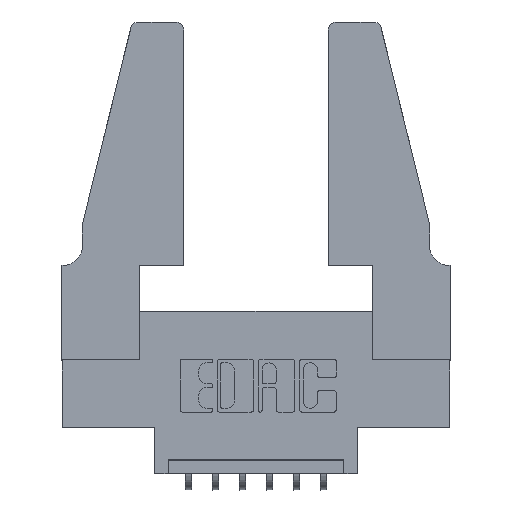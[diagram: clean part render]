
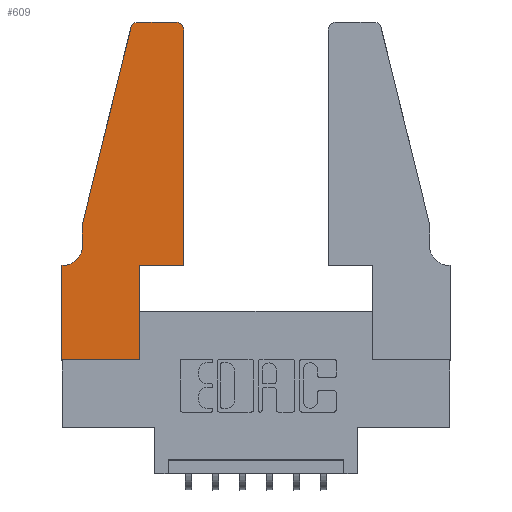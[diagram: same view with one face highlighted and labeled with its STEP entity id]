
A CAD part, top view. The second image highlights one B-rep face of the part: STEP entity #609.
In plain terms, the highlighted planar face has unit normal (0, 0, 1).
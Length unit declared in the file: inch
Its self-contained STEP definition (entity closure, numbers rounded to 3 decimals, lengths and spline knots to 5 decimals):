
#245 = EDGE_LOOP ( 'NONE', ( #11382, #3693, #6734, #3496, #2989, #1678, #5615, #2025, #9772, #2973, #2548, #9526 ) ) ;
#329 = VECTOR ( 'NONE', #9058, 39.37008 ) ;
#408 = LINE ( 'NONE', #6901, #4360 ) ;
#581 = CARTESIAN_POINT ( 'NONE',  ( 0.25487, 1.22718, 0.37 ) ) ;
#609 = ADVANCED_FACE ( 'NONE', ( #11190 ), #1291, .T. ) ;
#1291 = PLANE ( 'NONE',  #3030 ) ;
#1590 = VECTOR ( 'NONE', #2606, 39.37008 ) ;
#1604 = VERTEX_POINT ( 'NONE', #581 ) ;
#1656 = LINE ( 'NONE', #6720, #11586 ) ;
#1660 = CARTESIAN_POINT ( 'NONE',  ( 0.2605, 1.25, 0.37 ) ) ;
#1678 = ORIENTED_EDGE ( 'NONE', *, *, #3053, .T. ) ;
#1736 = LINE ( 'NONE', #8917, #1590 ) ;
#1852 = AXIS2_PLACEMENT_3D ( 'NONE', #11717, #9952, #9148 ) ;
#1861 = VERTEX_POINT ( 'NONE', #5412 ) ;
#2025 = ORIENTED_EDGE ( 'NONE', *, *, #3757, .T. ) ;
#2342 = EDGE_CURVE ( 'NONE', #1604, #7758, #8015, .T. ) ;
#2347 = CARTESIAN_POINT ( 'NONE',  ( 0.0755, 0.5, 0.37 ) ) ;
#2548 = ORIENTED_EDGE ( 'NONE', *, *, #7312, .T. ) ;
#2557 = CIRCLE ( 'NONE', #1852, 0.03 ) ;
#2606 = DIRECTION ( 'NONE',  ( 0., -1., 0. ) ) ;
#2674 = EDGE_CURVE ( 'NONE', #2938, #1604, #8461, .T. ) ;
#2734 = LINE ( 'NONE', #8519, #11380 ) ;
#2938 = VERTEX_POINT ( 'NONE', #3690 ) ;
#2939 = VECTOR ( 'NONE', #11372, 39.37008 ) ;
#2973 = ORIENTED_EDGE ( 'NONE', *, *, #9862, .T. ) ;
#2989 = ORIENTED_EDGE ( 'NONE', *, *, #3517, .T. ) ;
#3003 = DIRECTION ( 'NONE',  ( -1., 0., 0. ) ) ;
#3009 = DIRECTION ( 'NONE',  ( 0., 0., 1. ) ) ;
#3030 = AXIS2_PLACEMENT_3D ( 'NONE', #4083, #3009, #4995 ) ;
#3040 = DIRECTION ( 'NONE',  ( 0., -1., 0. ) ) ;
#3053 = EDGE_CURVE ( 'NONE', #10348, #5704, #9638, .T. ) ;
#3066 = DIRECTION ( 'NONE',  ( 1., 0., 0. ) ) ;
#3261 = LINE ( 'NONE', #4253, #11180 ) ;
#3496 = ORIENTED_EDGE ( 'NONE', *, *, #3575, .T. ) ;
#3517 = EDGE_CURVE ( 'NONE', #9332, #10348, #6536, .T. ) ;
#3575 = EDGE_CURVE ( 'NONE', #7758, #9332, #1656, .T. ) ;
#3690 = CARTESIAN_POINT ( 'NONE',  ( 0.284, 1.25, 0.37 ) ) ;
#3693 = ORIENTED_EDGE ( 'NONE', *, *, #2674, .T. ) ;
#3757 = EDGE_CURVE ( 'NONE', #11323, #10547, #408, .T. ) ;
#3964 = DIRECTION ( 'NONE',  ( 1., 0., 0. ) ) ;
#4083 = CARTESIAN_POINT ( 'NONE',  ( 0., 0.35, 0.37 ) ) ;
#4237 = CARTESIAN_POINT ( 'NONE',  ( 0., 0.35, 0.37 ) ) ;
#4253 = CARTESIAN_POINT ( 'NONE',  ( 0.2865, 0.35, 0.37 ) ) ;
#4360 = VECTOR ( 'NONE', #8670, 39.37008 ) ;
#4732 = DIRECTION ( 'NONE',  ( 0., 0., 1. ) ) ;
#4747 = DIRECTION ( 'NONE',  ( 0., 0., -1. ) ) ;
#4995 = DIRECTION ( 'NONE',  ( 1., 0., 0. ) ) ;
#5158 = VERTEX_POINT ( 'NONE', #5829 ) ;
#5159 = LINE ( 'NONE', #1660, #329 ) ;
#5283 = CARTESIAN_POINT ( 'NONE',  ( 0., 0., 0.37 ) ) ;
#5412 = CARTESIAN_POINT ( 'NONE',  ( 0.4505, 0.35, 0.37 ) ) ;
#5431 = CARTESIAN_POINT ( 'NONE',  ( 0.0755, 0.35, 0.37 ) ) ;
#5611 = CARTESIAN_POINT ( 'NONE',  ( 0.2865, 0., 0.37 ) ) ;
#5615 = ORIENTED_EDGE ( 'NONE', *, *, #6949, .T. ) ;
#5704 = VERTEX_POINT ( 'NONE', #4237 ) ;
#5829 = CARTESIAN_POINT ( 'NONE',  ( 0.4505, 1.22, 0.37 ) ) ;
#5961 = AXIS2_PLACEMENT_3D ( 'NONE', #10273, #4732, #3066 ) ;
#6022 = VECTOR ( 'NONE', #3964, 39.37008 ) ;
#6536 = CIRCLE ( 'NONE', #10624, 0.07 ) ;
#6635 = CARTESIAN_POINT ( 'NONE',  ( 0.2865, 0.35, 0.37 ) ) ;
#6720 = CARTESIAN_POINT ( 'NONE',  ( 0.0755, 0.5, 0.37 ) ) ;
#6734 = ORIENTED_EDGE ( 'NONE', *, *, #2342, .T. ) ;
#6901 = CARTESIAN_POINT ( 'NONE',  ( 0., 0., 0.37 ) ) ;
#6949 = EDGE_CURVE ( 'NONE', #5704, #11323, #1736, .T. ) ;
#7032 = CARTESIAN_POINT ( 'NONE',  ( 0.0755, 0.42, 0.37 ) ) ;
#7100 = VECTOR ( 'NONE', #9884, 39.37008 ) ;
#7123 = CARTESIAN_POINT ( 'NONE',  ( 0.4205, 1.25, 0.37 ) ) ;
#7312 = EDGE_CURVE ( 'NONE', #1861, #5158, #2734, .T. ) ;
#7758 = VERTEX_POINT ( 'NONE', #8430 ) ;
#8015 = LINE ( 'NONE', #2347, #2939 ) ;
#8128 = EDGE_CURVE ( 'NONE', #9403, #2938, #5159, .T. ) ;
#8336 = VERTEX_POINT ( 'NONE', #6635 ) ;
#8401 = LINE ( 'NONE', #11267, #6022 ) ;
#8430 = CARTESIAN_POINT ( 'NONE',  ( 0.0755, 0.5, 0.37 ) ) ;
#8461 = CIRCLE ( 'NONE', #5961, 0.03 ) ;
#8519 = CARTESIAN_POINT ( 'NONE',  ( 0.4505, 0.35, 0.37 ) ) ;
#8670 = DIRECTION ( 'NONE',  ( 1., 0., 0. ) ) ;
#8917 = CARTESIAN_POINT ( 'NONE',  ( 0., 0., 0.37 ) ) ;
#9058 = DIRECTION ( 'NONE',  ( -1., 0., 0. ) ) ;
#9148 = DIRECTION ( 'NONE',  ( 1., 0., 0. ) ) ;
#9332 = VERTEX_POINT ( 'NONE', #7032 ) ;
#9403 = VERTEX_POINT ( 'NONE', #7123 ) ;
#9436 = DIRECTION ( 'NONE',  ( 0., 1., 0. ) ) ;
#9526 = ORIENTED_EDGE ( 'NONE', *, *, #9686, .T. ) ;
#9638 = LINE ( 'NONE', #5431, #7100 ) ;
#9686 = EDGE_CURVE ( 'NONE', #5158, #9403, #2557, .T. ) ;
#9772 = ORIENTED_EDGE ( 'NONE', *, *, #11260, .T. ) ;
#9862 = EDGE_CURVE ( 'NONE', #8336, #1861, #8401, .T. ) ;
#9884 = DIRECTION ( 'NONE',  ( -1., 0., 0. ) ) ;
#9952 = DIRECTION ( 'NONE',  ( 0., 0., 1. ) ) ;
#10160 = CARTESIAN_POINT ( 'NONE',  ( 0.0055, 0.42, 0.37 ) ) ;
#10273 = CARTESIAN_POINT ( 'NONE',  ( 0.284, 1.22, 0.37 ) ) ;
#10348 = VERTEX_POINT ( 'NONE', #10565 ) ;
#10547 = VERTEX_POINT ( 'NONE', #5611 ) ;
#10565 = CARTESIAN_POINT ( 'NONE',  ( 0.0055, 0.35, 0.37 ) ) ;
#10624 = AXIS2_PLACEMENT_3D ( 'NONE', #10160, #4747, #3003 ) ;
#10812 = DIRECTION ( 'NONE',  ( 0., 1., 0. ) ) ;
#11180 = VECTOR ( 'NONE', #10812, 39.37008 ) ;
#11190 = FACE_OUTER_BOUND ( 'NONE', #245, .T. ) ;
#11260 = EDGE_CURVE ( 'NONE', #10547, #8336, #3261, .T. ) ;
#11267 = CARTESIAN_POINT ( 'NONE',  ( 0.4505, 0.35, 0.37 ) ) ;
#11323 = VERTEX_POINT ( 'NONE', #5283 ) ;
#11372 = DIRECTION ( 'NONE',  ( -0.239, -0.971, 0. ) ) ;
#11380 = VECTOR ( 'NONE', #9436, 39.37008 ) ;
#11382 = ORIENTED_EDGE ( 'NONE', *, *, #8128, .T. ) ;
#11586 = VECTOR ( 'NONE', #3040, 39.37008 ) ;
#11717 = CARTESIAN_POINT ( 'NONE',  ( 0.4205, 1.22, 0.37 ) ) ;
